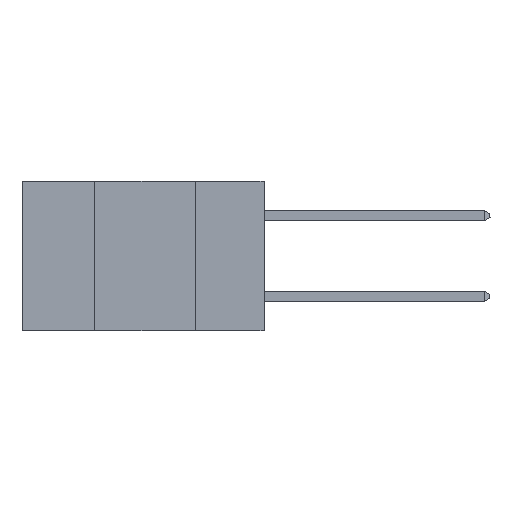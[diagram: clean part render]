
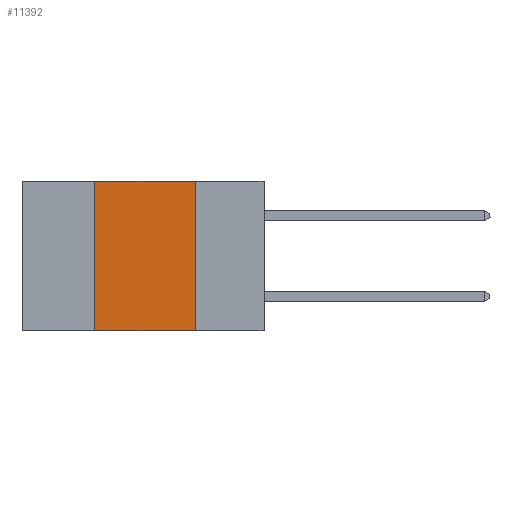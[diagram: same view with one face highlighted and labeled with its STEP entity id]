
A CAD part, left-side view. The second image highlights one B-rep face of the part: STEP entity #11392.
In plain terms, the highlighted planar face has unit normal (-1, 0, 0).
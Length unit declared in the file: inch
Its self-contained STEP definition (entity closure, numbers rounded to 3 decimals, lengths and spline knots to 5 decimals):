
#394 = ORIENTED_EDGE ( 'NONE', *, *, #14660, .F. ) ;
#1148 = LINE ( 'NONE', #11784, #5035 ) ;
#2592 = ORIENTED_EDGE ( 'NONE', *, *, #9422, .T. ) ;
#2895 = FACE_OUTER_BOUND ( 'NONE', #15334, .T. ) ;
#4199 = DIRECTION ( 'NONE',  ( 0., -1., 0. ) ) ;
#4255 = VERTEX_POINT ( 'NONE', #8191 ) ;
#4257 = CARTESIAN_POINT ( 'NONE',  ( 0., 0.6, 0. ) ) ;
#5035 = VECTOR ( 'NONE', #13345, 39.37008 ) ;
#5362 = CARTESIAN_POINT ( 'NONE',  ( 0., 0.6, 0. ) ) ;
#5525 = DIRECTION ( 'NONE',  ( 0., -1., 0. ) ) ;
#5749 = VECTOR ( 'NONE', #4199, 39.37008 ) ;
#5792 = VERTEX_POINT ( 'NONE', #9444 ) ;
#6171 = ORIENTED_EDGE ( 'NONE', *, *, #14622, .F. ) ;
#6632 = VERTEX_POINT ( 'NONE', #16878 ) ;
#8112 = LINE ( 'NONE', #9545, #13690 ) ;
#8191 = CARTESIAN_POINT ( 'NONE',  ( 0., 0.17, 0. ) ) ;
#9422 = EDGE_CURVE ( 'NONE', #6632, #5792, #9936, .T. ) ;
#9444 = CARTESIAN_POINT ( 'NONE',  ( 0., 0.17, -0.37 ) ) ;
#9545 = CARTESIAN_POINT ( 'NONE',  ( 0., 0.42, 0. ) ) ;
#9936 = LINE ( 'NONE', #14647, #13238 ) ;
#10540 = DIRECTION ( 'NONE',  ( 1., 0., 0. ) ) ;
#11392 = ADVANCED_FACE ( 'NONE', ( #2895 ), #14594, .F. ) ;
#11464 = EDGE_CURVE ( 'NONE', #14428, #4255, #16087, .T. ) ;
#11681 = CARTESIAN_POINT ( 'NONE',  ( 0., 0.42, 0. ) ) ;
#11784 = CARTESIAN_POINT ( 'NONE',  ( 0., 0.17, 0. ) ) ;
#13047 = ORIENTED_EDGE ( 'NONE', *, *, #11464, .F. ) ;
#13238 = VECTOR ( 'NONE', #5525, 39.37008 ) ;
#13345 = DIRECTION ( 'NONE',  ( 0., 0., -1. ) ) ;
#13690 = VECTOR ( 'NONE', #14958, 39.37008 ) ;
#14425 = DIRECTION ( 'NONE',  ( 0., 0., -1. ) ) ;
#14428 = VERTEX_POINT ( 'NONE', #11681 ) ;
#14594 = PLANE ( 'NONE',  #16283 ) ;
#14622 = EDGE_CURVE ( 'NONE', #4255, #5792, #1148, .T. ) ;
#14647 = CARTESIAN_POINT ( 'NONE',  ( 0., 0.6, -0.37 ) ) ;
#14660 = EDGE_CURVE ( 'NONE', #6632, #14428, #8112, .T. ) ;
#14958 = DIRECTION ( 'NONE',  ( 0., 0., 1. ) ) ;
#15334 = EDGE_LOOP ( 'NONE', ( #6171, #13047, #394, #2592 ) ) ;
#16087 = LINE ( 'NONE', #4257, #5749 ) ;
#16283 = AXIS2_PLACEMENT_3D ( 'NONE', #5362, #10540, #14425 ) ;
#16878 = CARTESIAN_POINT ( 'NONE',  ( 0., 0.42, -0.37 ) ) ;
